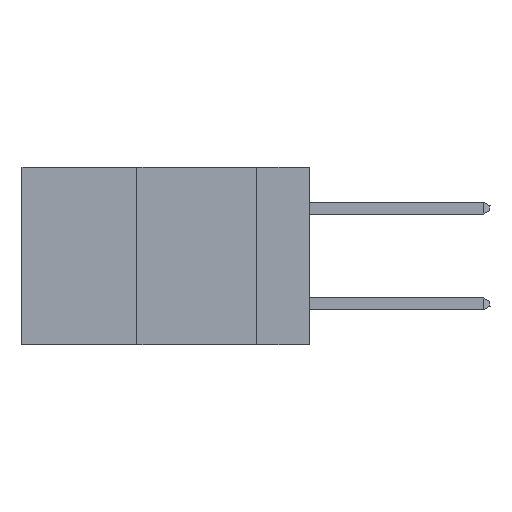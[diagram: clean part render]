
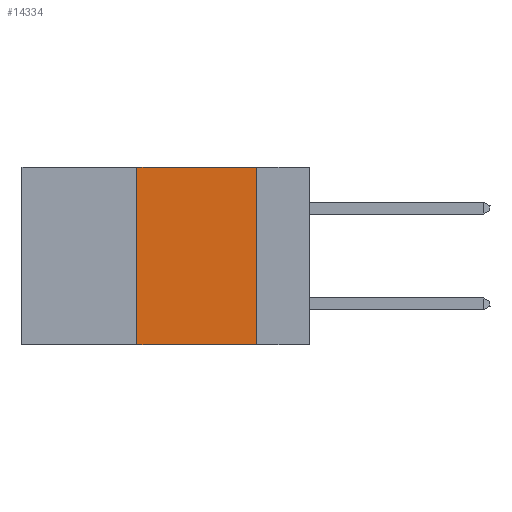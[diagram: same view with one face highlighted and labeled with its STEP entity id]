
A CAD part, left-side view. The second image highlights one B-rep face of the part: STEP entity #14334.
In plain terms, the highlighted planar face has unit normal (-1, 0, 0).
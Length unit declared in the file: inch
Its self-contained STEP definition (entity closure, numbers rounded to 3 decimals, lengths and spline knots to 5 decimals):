
#1303 = DIRECTION ( 'NONE',  ( 0., 0., -1. ) ) ;
#1725 = VERTEX_POINT ( 'NONE', #31935 ) ;
#2072 = VECTOR ( 'NONE', #7502, 39.37008 ) ;
#3201 = VECTOR ( 'NONE', #8783, 39.37008 ) ;
#4841 = EDGE_CURVE ( 'NONE', #1725, #27005, #23398, .T. ) ;
#7502 = DIRECTION ( 'NONE',  ( 0., -1., 0. ) ) ;
#8783 = DIRECTION ( 'NONE',  ( 0., 0., -1. ) ) ;
#8884 = CARTESIAN_POINT ( 'NONE',  ( 0., 0.36, 0. ) ) ;
#9478 = DIRECTION ( 'NONE',  ( 0., 0., 1. ) ) ;
#9538 = ORIENTED_EDGE ( 'NONE', *, *, #9801, .F. ) ;
#9801 = EDGE_CURVE ( 'NONE', #27005, #13352, #18490, .T. ) ;
#11402 = VECTOR ( 'NONE', #9478, 39.37008 ) ;
#12075 = DIRECTION ( 'NONE',  ( 0., -1., 0. ) ) ;
#13352 = VERTEX_POINT ( 'NONE', #20965 ) ;
#14206 = PLANE ( 'NONE',  #17518 ) ;
#14334 = ADVANCED_FACE ( 'NONE', ( #28055 ), #14206, .F. ) ;
#16930 = DIRECTION ( 'NONE',  ( 1., 0., 0. ) ) ;
#17518 = AXIS2_PLACEMENT_3D ( 'NONE', #31834, #16930, #1303 ) ;
#18490 = LINE ( 'NONE', #22279, #24306 ) ;
#19803 = CARTESIAN_POINT ( 'NONE',  ( 0., 0.36, 0. ) ) ;
#20965 = CARTESIAN_POINT ( 'NONE',  ( 0., 0.11, 0. ) ) ;
#21506 = EDGE_LOOP ( 'NONE', ( #23564, #9538, #22823, #28215 ) ) ;
#21647 = CARTESIAN_POINT ( 'NONE',  ( 0., 0.11, 0. ) ) ;
#21688 = EDGE_CURVE ( 'NONE', #1725, #30806, #22661, .T. ) ;
#22279 = CARTESIAN_POINT ( 'NONE',  ( 0., 0.6, 0. ) ) ;
#22661 = LINE ( 'NONE', #25386, #2072 ) ;
#22823 = ORIENTED_EDGE ( 'NONE', *, *, #4841, .F. ) ;
#23043 = CARTESIAN_POINT ( 'NONE',  ( 0., 0.11, -0.37 ) ) ;
#23157 = EDGE_CURVE ( 'NONE', #13352, #30806, #29500, .T. ) ;
#23398 = LINE ( 'NONE', #19803, #11402 ) ;
#23564 = ORIENTED_EDGE ( 'NONE', *, *, #23157, .F. ) ;
#24306 = VECTOR ( 'NONE', #12075, 39.37008 ) ;
#25386 = CARTESIAN_POINT ( 'NONE',  ( 0., 0.6, -0.37 ) ) ;
#27005 = VERTEX_POINT ( 'NONE', #8884 ) ;
#28055 = FACE_OUTER_BOUND ( 'NONE', #21506, .T. ) ;
#28215 = ORIENTED_EDGE ( 'NONE', *, *, #21688, .T. ) ;
#29500 = LINE ( 'NONE', #21647, #3201 ) ;
#30806 = VERTEX_POINT ( 'NONE', #23043 ) ;
#31834 = CARTESIAN_POINT ( 'NONE',  ( 0., 0.6, 0. ) ) ;
#31935 = CARTESIAN_POINT ( 'NONE',  ( 0., 0.36, -0.37 ) ) ;
